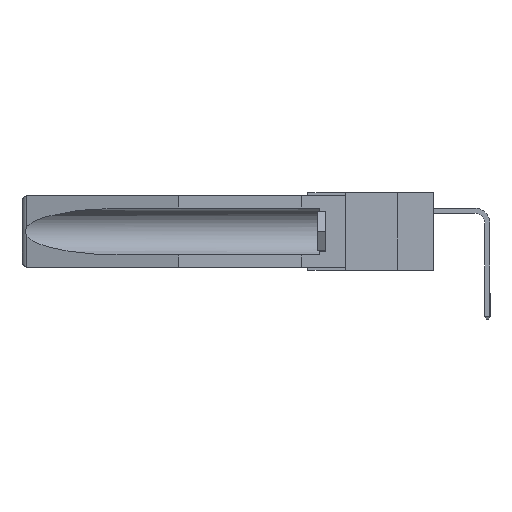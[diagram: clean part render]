
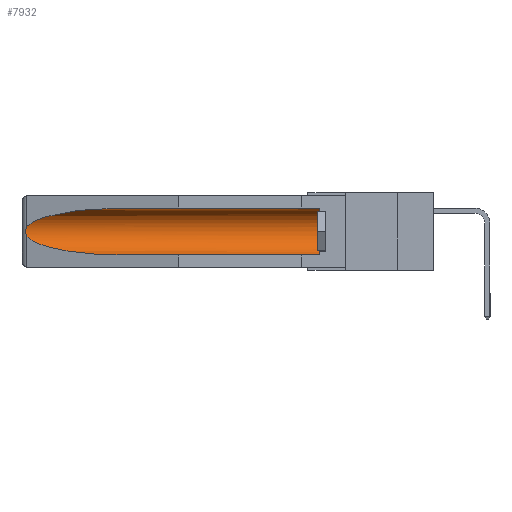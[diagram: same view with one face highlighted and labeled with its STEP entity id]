
A CAD part, left-side view. The second image highlights one B-rep face of the part: STEP entity #7932.
In plain terms, the highlighted cylindrical face has radius 2.857 mm (diameter 5.715 mm), a partial arc.
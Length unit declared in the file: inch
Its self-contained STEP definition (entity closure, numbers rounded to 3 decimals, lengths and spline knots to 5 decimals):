
#73 = EDGE_CURVE ( 'NONE', #5105, #12058, #9468, .T. ) ;
#117 =( BOUNDED_CURVE ( )  B_SPLINE_CURVE ( 3, ( #20452, #12463, #20659, #4197 ),
 .UNSPECIFIED., .F., .F. ) 
 B_SPLINE_CURVE_WITH_KNOTS ( ( 4, 4 ),
 ( 0.1948, 1.5708 ),
 .UNSPECIFIED. ) 
 CURVE ( )  GEOMETRIC_REPRESENTATION_ITEM ( )  RATIONAL_B_SPLINE_CURVE ( ( 1., 0.848, 0.848, 1. ) ) 
 REPRESENTATION_ITEM ( '' )  );
#765 =( BOUNDED_CURVE ( )  B_SPLINE_CURVE ( 3, ( #875, #18768, #12381, #5980 ),
 .UNSPECIFIED., .F., .T. ) 
 B_SPLINE_CURVE_WITH_KNOTS ( ( 4, 4 ),
 ( 4.71239, 6.08839 ),
 .UNSPECIFIED. ) 
 CURVE ( )  GEOMETRIC_REPRESENTATION_ITEM ( )  RATIONAL_B_SPLINE_CURVE ( ( 1., 0.848, 0.848, 1. ) ) 
 REPRESENTATION_ITEM ( '' )  );
#875 = CARTESIAN_POINT ( 'NONE',  ( 0.155, 1.07973, -0.059 ) ) ;
#1140 = ORIENTED_EDGE ( 'NONE', *, *, #73, .F. ) ;
#1985 = FACE_OUTER_BOUND ( 'NONE', #18134, .T. ) ;
#2141 = CARTESIAN_POINT ( 'NONE',  ( 0.155, 1.07973, -0.059 ) ) ;
#2419 = CARTESIAN_POINT ( 'NONE',  ( 0.26537, 1.52718, -0.14972 ) ) ;
#2929 = ORIENTED_EDGE ( 'NONE', *, *, #4408, .T. ) ;
#3630 = EDGE_CURVE ( 'NONE', #16367, #11246, #765, .T. ) ;
#3953 = CARTESIAN_POINT ( 'NONE',  ( 0.2673, 1.5327, -0.16383 ) ) ;
#4197 = CARTESIAN_POINT ( 'NONE',  ( 0.155, 1.07973, -0.284 ) ) ;
#4243 = ORIENTED_EDGE ( 'NONE', *, *, #3630, .T. ) ;
#4408 = EDGE_CURVE ( 'NONE', #11246, #9009, #11420, .T. ) ;
#4566 = VECTOR ( 'NONE', #7697, 39.37008 ) ;
#4856 = CARTESIAN_POINT ( 'NONE',  ( 0.155, 1.07973, -0.284 ) ) ;
#5105 = VERTEX_POINT ( 'NONE', #10203 ) ;
#5980 = CARTESIAN_POINT ( 'NONE',  ( 0.26537, 1.52718, -0.14972 ) ) ;
#6687 = CARTESIAN_POINT ( 'NONE',  ( 0.155, 0.126, -0.059 ) ) ;
#6879 = DIRECTION ( 'NONE',  ( 0., -1., 0. ) ) ;
#7174 = EDGE_CURVE ( 'NONE', #20027, #16367, #18009, .T. ) ;
#7329 = CIRCLE ( 'NONE', #17879, 0.1125 ) ;
#7697 = DIRECTION ( 'NONE',  ( 0., 1., 0. ) ) ;
#7932 = ADVANCED_FACE ( 'NONE', ( #1985 ), #12875, .F. ) ;
#8559 = EDGE_CURVE ( 'NONE', #9009, #12058, #117, .T. ) ;
#8675 = ORIENTED_EDGE ( 'NONE', *, *, #7174, .T. ) ;
#9009 = VERTEX_POINT ( 'NONE', #20584 ) ;
#9374 = CARTESIAN_POINT ( 'NONE',  ( 0.155, -0.30754, -0.284 ) ) ;
#9468 = LINE ( 'NONE', #9374, #13036 ) ;
#9755 = AXIS2_PLACEMENT_3D ( 'NONE', #12575, #19094, #12932 ) ;
#9877 = DIRECTION ( 'NONE',  ( 0., 0., 1. ) ) ;
#10203 = CARTESIAN_POINT ( 'NONE',  ( 0.155, 0.126, -0.284 ) ) ;
#10379 = ORIENTED_EDGE ( 'NONE', *, *, #8559, .T. ) ;
#11057 = DIRECTION ( 'NONE',  ( 0., 1., 0. ) ) ;
#11246 = VERTEX_POINT ( 'NONE', #2419 ) ;
#11420 = B_SPLINE_CURVE_WITH_KNOTS ( 'NONE', 3,
 ( #12012, #18340, #18480, #3953, #13438, #15133, #20029, #11786, #13637, #19816 ),
 .UNSPECIFIED., .F., .F.,
 ( 4, 2, 2, 2, 4 ),
 ( 0., 0.00029, 0.00058, 0.00087, 0.00117 ),
 .UNSPECIFIED. ) ;
#11786 = CARTESIAN_POINT ( 'NONE',  ( 0.26655, 1.53094, -0.18657 ) ) ;
#12012 = CARTESIAN_POINT ( 'NONE',  ( 0.26537, 1.52718, -0.14972 ) ) ;
#12058 = VERTEX_POINT ( 'NONE', #4856 ) ;
#12224 = EDGE_CURVE ( 'NONE', #5105, #20027, #7329, .T. ) ;
#12381 = CARTESIAN_POINT ( 'NONE',  ( 0.25451, 1.48313, -0.09465 ) ) ;
#12463 = CARTESIAN_POINT ( 'NONE',  ( 0.25451, 1.48313, -0.24835 ) ) ;
#12541 = CARTESIAN_POINT ( 'NONE',  ( 0.155, -0.30754, -0.059 ) ) ;
#12575 = CARTESIAN_POINT ( 'NONE',  ( 0.155, -0.30754, -0.1715 ) ) ;
#12875 = CYLINDRICAL_SURFACE ( 'NONE', #9755, 0.1125 ) ;
#12932 = DIRECTION ( 'NONE',  ( 0., 0., 1. ) ) ;
#13036 = VECTOR ( 'NONE', #11057, 39.37008 ) ;
#13438 = CARTESIAN_POINT ( 'NONE',  ( 0.2675, 1.53308, -0.16763 ) ) ;
#13637 = CARTESIAN_POINT ( 'NONE',  ( 0.26597, 1.5296, -0.19026 ) ) ;
#15133 = CARTESIAN_POINT ( 'NONE',  ( 0.2675, 1.53308, -0.17534 ) ) ;
#15517 = ORIENTED_EDGE ( 'NONE', *, *, #12224, .T. ) ;
#16367 = VERTEX_POINT ( 'NONE', #2141 ) ;
#17879 = AXIS2_PLACEMENT_3D ( 'NONE', #19582, #6879, #9877 ) ;
#18009 = LINE ( 'NONE', #12541, #4566 ) ;
#18134 = EDGE_LOOP ( 'NONE', ( #4243, #2929, #10379, #1140, #15517, #8675 ) ) ;
#18340 = CARTESIAN_POINT ( 'NONE',  ( 0.26597, 1.52961, -0.15275 ) ) ;
#18480 = CARTESIAN_POINT ( 'NONE',  ( 0.26654, 1.53092, -0.15636 ) ) ;
#18768 = CARTESIAN_POINT ( 'NONE',  ( 0.21114, 1.30732, -0.059 ) ) ;
#19094 = DIRECTION ( 'NONE',  ( 0., 1., 0. ) ) ;
#19582 = CARTESIAN_POINT ( 'NONE',  ( 0.155, 0.126, -0.1715 ) ) ;
#19816 = CARTESIAN_POINT ( 'NONE',  ( 0.26537, 1.52718, -0.19328 ) ) ;
#20027 = VERTEX_POINT ( 'NONE', #6687 ) ;
#20029 = CARTESIAN_POINT ( 'NONE',  ( 0.2673, 1.53269, -0.17917 ) ) ;
#20452 = CARTESIAN_POINT ( 'NONE',  ( 0.26537, 1.52718, -0.19328 ) ) ;
#20584 = CARTESIAN_POINT ( 'NONE',  ( 0.26537, 1.52718, -0.19328 ) ) ;
#20659 = CARTESIAN_POINT ( 'NONE',  ( 0.21114, 1.30732, -0.284 ) ) ;
